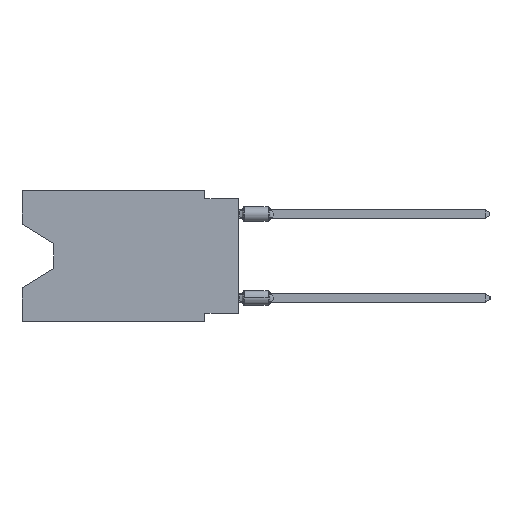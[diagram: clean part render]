
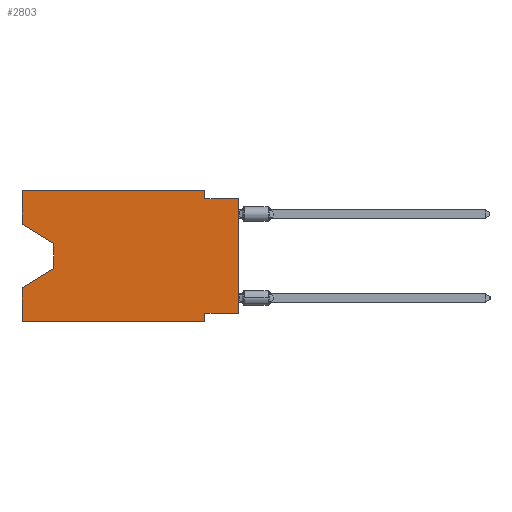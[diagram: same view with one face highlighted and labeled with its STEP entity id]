
A CAD part, left-side view. The second image highlights one B-rep face of the part: STEP entity #2803.
In plain terms, the highlighted planar face has unit normal (-1, 0, 0).
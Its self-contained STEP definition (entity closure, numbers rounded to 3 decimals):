
#1243 = VECTOR ( 'NONE', #20174, 1000. ) ;
#1373 = EDGE_CURVE ( 'NONE', #5365, #44123, #38785, .T. ) ;
#1956 = VECTOR ( 'NONE', #50898, 1000. ) ;
#2395 = CARTESIAN_POINT ( 'NONE',  ( 0., 16.383, 0. ) ) ;
#2803 = ADVANCED_FACE ( 'NONE', ( #38082 ), #57987, .F. ) ;
#2986 = CARTESIAN_POINT ( 'NONE',  ( 0., 16.383, 0. ) ) ;
#3172 = LINE ( 'NONE', #7973, #36992 ) ;
#3941 = LINE ( 'NONE', #2986, #35717 ) ;
#4006 = VECTOR ( 'NONE', #58695, 1000. ) ;
#4116 = VECTOR ( 'NONE', #29212, 1000. ) ;
#4388 = DIRECTION ( 'NONE',  ( 1., 0., 0. ) ) ;
#5365 = VERTEX_POINT ( 'NONE', #5730 ) ;
#5730 = CARTESIAN_POINT ( 'NONE',  ( 0., 16.383, -9.906 ) ) ;
#7210 = ORIENTED_EDGE ( 'NONE', *, *, #1373, .F. ) ;
#7373 = VECTOR ( 'NONE', #53314, 1000. ) ;
#7450 = VECTOR ( 'NONE', #8808, 1000. ) ;
#7973 = CARTESIAN_POINT ( 'NONE',  ( 0., 16.383, -9.906 ) ) ;
#8808 = DIRECTION ( 'NONE',  ( 0., -1., 0. ) ) ;
#10188 = CARTESIAN_POINT ( 'NONE',  ( 0., 13.97, -5.893 ) ) ;
#12206 = ORIENTED_EDGE ( 'NONE', *, *, #38558, .F. ) ;
#12447 = EDGE_CURVE ( 'NONE', #29958, #57719, #40949, .T. ) ;
#12923 = EDGE_CURVE ( 'NONE', #19804, #48845, #53945, .T. ) ;
#14494 = ORIENTED_EDGE ( 'NONE', *, *, #16277, .F. ) ;
#14841 = EDGE_CURVE ( 'NONE', #53918, #29958, #33888, .T. ) ;
#15562 = EDGE_CURVE ( 'NONE', #59272, #26670, #34620, .T. ) ;
#15885 = CARTESIAN_POINT ( 'NONE',  ( 0., 0., -9.271 ) ) ;
#16103 = ORIENTED_EDGE ( 'NONE', *, *, #39083, .T. ) ;
#16277 = EDGE_CURVE ( 'NONE', #48845, #19002, #57282, .T. ) ;
#16530 = CARTESIAN_POINT ( 'NONE',  ( 0., 13.97, -5.893 ) ) ;
#17745 = CARTESIAN_POINT ( 'NONE',  ( 0., 2.54, -9.271 ) ) ;
#18185 = DIRECTION ( 'NONE',  ( 0., 0., -1. ) ) ;
#18700 = DIRECTION ( 'NONE',  ( 0., -1., 0. ) ) ;
#19002 = VERTEX_POINT ( 'NONE', #34708 ) ;
#19804 = VERTEX_POINT ( 'NONE', #29979 ) ;
#20131 = LINE ( 'NONE', #10188, #54202 ) ;
#20174 = DIRECTION ( 'NONE',  ( 0., 0., -1. ) ) ;
#20629 = EDGE_CURVE ( 'NONE', #20814, #59272, #39469, .T. ) ;
#20814 = VERTEX_POINT ( 'NONE', #38928 ) ;
#22095 = CARTESIAN_POINT ( 'NONE',  ( 0., 2.54, -0.635 ) ) ;
#22585 = ORIENTED_EDGE ( 'NONE', *, *, #25630, .F. ) ;
#22806 = CARTESIAN_POINT ( 'NONE',  ( 0., 16.383, 0. ) ) ;
#25534 = LINE ( 'NONE', #41549, #27779 ) ;
#25630 = EDGE_CURVE ( 'NONE', #20814, #50974, #33712, .T. ) ;
#26670 = VERTEX_POINT ( 'NONE', #16530 ) ;
#26844 = EDGE_CURVE ( 'NONE', #53918, #19002, #25534, .T. ) ;
#27779 = VECTOR ( 'NONE', #45105, 1000. ) ;
#28309 = ORIENTED_EDGE ( 'NONE', *, *, #12447, .F. ) ;
#29212 = DIRECTION ( 'NONE',  ( 0., 0., 1. ) ) ;
#29394 = DIRECTION ( 'NONE',  ( 0., 1., 0. ) ) ;
#29432 = ORIENTED_EDGE ( 'NONE', *, *, #15562, .T. ) ;
#29958 = VERTEX_POINT ( 'NONE', #17745 ) ;
#29979 = CARTESIAN_POINT ( 'NONE',  ( 0., 2.54, 0. ) ) ;
#31289 = ORIENTED_EDGE ( 'NONE', *, *, #26844, .T. ) ;
#33712 = LINE ( 'NONE', #22806, #4116 ) ;
#33888 = LINE ( 'NONE', #53479, #50389 ) ;
#34620 = LINE ( 'NONE', #59353, #1243 ) ;
#34708 = CARTESIAN_POINT ( 'NONE',  ( 0., 0., -0.635 ) ) ;
#34894 = DIRECTION ( 'NONE',  ( 0., 0.855, -0.519 ) ) ;
#35717 = VECTOR ( 'NONE', #18700, 1000. ) ;
#36992 = VECTOR ( 'NONE', #56469, 1000. ) ;
#38082 = FACE_OUTER_BOUND ( 'NONE', #49633, .T. ) ;
#38558 = EDGE_CURVE ( 'NONE', #50974, #19804, #3941, .T. ) ;
#38785 = LINE ( 'NONE', #39430, #4006 ) ;
#38928 = CARTESIAN_POINT ( 'NONE',  ( 0., 16.383, -2.546 ) ) ;
#39083 = EDGE_CURVE ( 'NONE', #26670, #44123, #20131, .T. ) ;
#39430 = CARTESIAN_POINT ( 'NONE',  ( 0., 16.383, 0. ) ) ;
#39469 = LINE ( 'NONE', #43959, #63326 ) ;
#40850 = ORIENTED_EDGE ( 'NONE', *, *, #12923, .F. ) ;
#40949 = LINE ( 'NONE', #55728, #1956 ) ;
#41549 = CARTESIAN_POINT ( 'NONE',  ( 0., 0., 0. ) ) ;
#42347 = ORIENTED_EDGE ( 'NONE', *, *, #45483, .T. ) ;
#42511 = CARTESIAN_POINT ( 'NONE',  ( 0., 0., -0.635 ) ) ;
#43280 = CARTESIAN_POINT ( 'NONE',  ( 0., 16.383, -7.36 ) ) ;
#43548 = CARTESIAN_POINT ( 'NONE',  ( 0., 2.54, -9.906 ) ) ;
#43959 = CARTESIAN_POINT ( 'NONE',  ( 0., 16.383, -2.546 ) ) ;
#44013 = ORIENTED_EDGE ( 'NONE', *, *, #14841, .F. ) ;
#44123 = VERTEX_POINT ( 'NONE', #43280 ) ;
#45105 = DIRECTION ( 'NONE',  ( 0., 0., 1. ) ) ;
#45319 = ORIENTED_EDGE ( 'NONE', *, *, #20629, .T. ) ;
#45483 = EDGE_CURVE ( 'NONE', #5365, #57719, #3172, .T. ) ;
#47076 = CARTESIAN_POINT ( 'NONE',  ( 0., 16.383, 0. ) ) ;
#48845 = VERTEX_POINT ( 'NONE', #22095 ) ;
#49117 = CARTESIAN_POINT ( 'NONE',  ( 0., 2.54, 0. ) ) ;
#49633 = EDGE_LOOP ( 'NONE', ( #45319, #29432, #16103, #7210, #42347, #28309, #44013, #31289, #14494, #40850, #12206, #22585 ) ) ;
#50389 = VECTOR ( 'NONE', #29394, 1000. ) ;
#50898 = DIRECTION ( 'NONE',  ( 0., 0., -1. ) ) ;
#50974 = VERTEX_POINT ( 'NONE', #2395 ) ;
#53314 = DIRECTION ( 'NONE',  ( 0., 0., -1. ) ) ;
#53479 = CARTESIAN_POINT ( 'NONE',  ( 0., 0., -9.271 ) ) ;
#53918 = VERTEX_POINT ( 'NONE', #15885 ) ;
#53945 = LINE ( 'NONE', #49117, #7373 ) ;
#54202 = VECTOR ( 'NONE', #34894, 1000. ) ;
#55728 = CARTESIAN_POINT ( 'NONE',  ( 0., 2.54, -9.906 ) ) ;
#56131 = CARTESIAN_POINT ( 'NONE',  ( 0., 13.97, -4.013 ) ) ;
#56469 = DIRECTION ( 'NONE',  ( 0., -1., 0. ) ) ;
#57282 = LINE ( 'NONE', #42511, #7450 ) ;
#57719 = VERTEX_POINT ( 'NONE', #43548 ) ;
#57987 = PLANE ( 'NONE',  #62547 ) ;
#58412 = DIRECTION ( 'NONE',  ( 0., -0.855, -0.519 ) ) ;
#58695 = DIRECTION ( 'NONE',  ( 0., 0., 1. ) ) ;
#59272 = VERTEX_POINT ( 'NONE', #56131 ) ;
#59353 = CARTESIAN_POINT ( 'NONE',  ( 0., 13.97, -4.013 ) ) ;
#62547 = AXIS2_PLACEMENT_3D ( 'NONE', #47076, #4388, #18185 ) ;
#63326 = VECTOR ( 'NONE', #58412, 1000. ) ;
